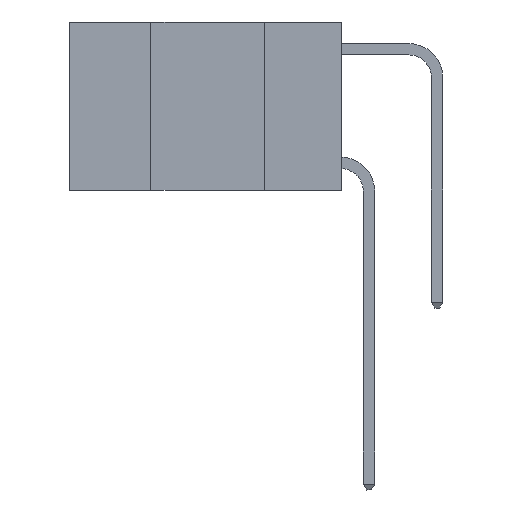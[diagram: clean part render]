
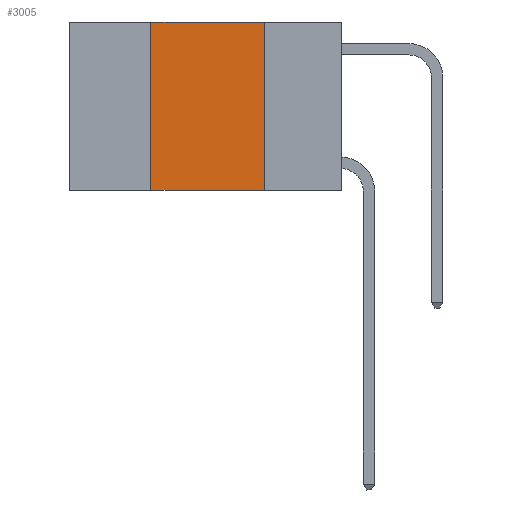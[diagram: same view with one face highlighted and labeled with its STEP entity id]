
A CAD part, left-side view. The second image highlights one B-rep face of the part: STEP entity #3005.
In plain terms, the highlighted planar face has unit normal (-1, 0, 0).
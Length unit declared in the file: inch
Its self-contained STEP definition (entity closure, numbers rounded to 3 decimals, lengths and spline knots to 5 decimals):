
#12 = CARTESIAN_POINT ( 'NONE',  ( 0., 0.42, -0.37 ) ) ;
#204 = PLANE ( 'NONE',  #4812 ) ;
#1096 = DIRECTION ( 'NONE',  ( 1., 0., 0. ) ) ;
#1218 = CARTESIAN_POINT ( 'NONE',  ( 0., 0.17, 0. ) ) ;
#1707 = EDGE_LOOP ( 'NONE', ( #3711, #5863, #8050, #8290 ) ) ;
#1831 = CARTESIAN_POINT ( 'NONE',  ( 0., 0.6, 0. ) ) ;
#1855 = VERTEX_POINT ( 'NONE', #2280 ) ;
#2106 = VECTOR ( 'NONE', #8507, 39.37008 ) ;
#2119 = LINE ( 'NONE', #6289, #6131 ) ;
#2280 = CARTESIAN_POINT ( 'NONE',  ( 0., 0.17, 0. ) ) ;
#2356 = CARTESIAN_POINT ( 'NONE',  ( 0., 0.17, -0.37 ) ) ;
#2964 = LINE ( 'NONE', #7729, #6479 ) ;
#3005 = ADVANCED_FACE ( 'NONE', ( #7162 ), #204, .F. ) ;
#3084 = DIRECTION ( 'NONE',  ( 0., 0., 1. ) ) ;
#3168 = CARTESIAN_POINT ( 'NONE',  ( 0., 0.42, 0. ) ) ;
#3410 = DIRECTION ( 'NONE',  ( 0., 0., -1. ) ) ;
#3656 = VERTEX_POINT ( 'NONE', #12 ) ;
#3711 = ORIENTED_EDGE ( 'NONE', *, *, #8720, .F. ) ;
#4069 = EDGE_CURVE ( 'NONE', #5136, #1855, #9206, .T. ) ;
#4812 = AXIS2_PLACEMENT_3D ( 'NONE', #10345, #1096, #3410 ) ;
#5136 = VERTEX_POINT ( 'NONE', #3168 ) ;
#5298 = DIRECTION ( 'NONE',  ( 0., -1., 0. ) ) ;
#5514 = DIRECTION ( 'NONE',  ( 0., -1., 0. ) ) ;
#5863 = ORIENTED_EDGE ( 'NONE', *, *, #4069, .F. ) ;
#6131 = VECTOR ( 'NONE', #3084, 39.37008 ) ;
#6289 = CARTESIAN_POINT ( 'NONE',  ( 0., 0.42, 0. ) ) ;
#6479 = VECTOR ( 'NONE', #5298, 39.37008 ) ;
#6621 = LINE ( 'NONE', #1218, #2106 ) ;
#7162 = FACE_OUTER_BOUND ( 'NONE', #1707, .T. ) ;
#7289 = VERTEX_POINT ( 'NONE', #2356 ) ;
#7729 = CARTESIAN_POINT ( 'NONE',  ( 0., 0.6, -0.37 ) ) ;
#8050 = ORIENTED_EDGE ( 'NONE', *, *, #8231, .F. ) ;
#8231 = EDGE_CURVE ( 'NONE', #3656, #5136, #2119, .T. ) ;
#8290 = ORIENTED_EDGE ( 'NONE', *, *, #10340, .T. ) ;
#8507 = DIRECTION ( 'NONE',  ( 0., 0., -1. ) ) ;
#8720 = EDGE_CURVE ( 'NONE', #1855, #7289, #6621, .T. ) ;
#9206 = LINE ( 'NONE', #1831, #9456 ) ;
#9456 = VECTOR ( 'NONE', #5514, 39.37008 ) ;
#10340 = EDGE_CURVE ( 'NONE', #3656, #7289, #2964, .T. ) ;
#10345 = CARTESIAN_POINT ( 'NONE',  ( 0., 0.6, 0. ) ) ;
